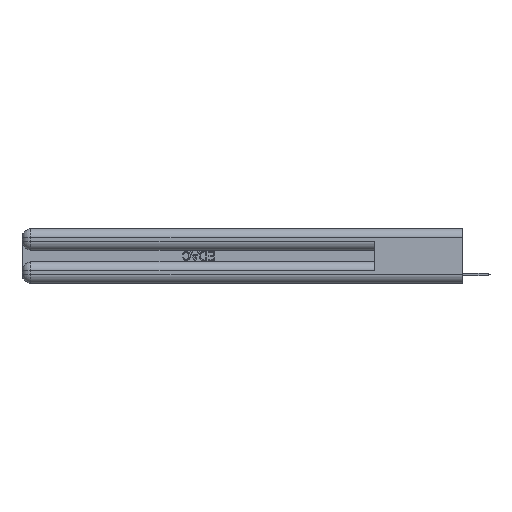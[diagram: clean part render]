
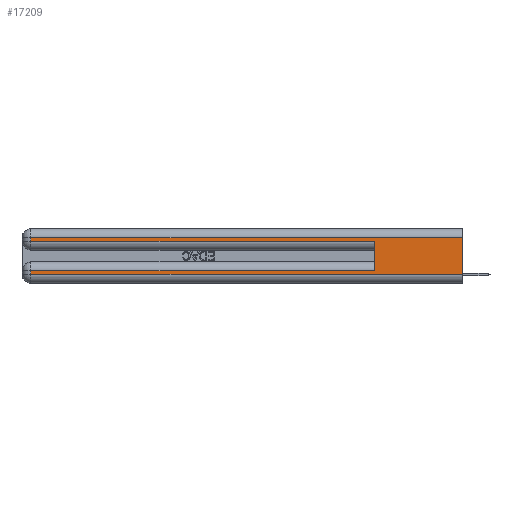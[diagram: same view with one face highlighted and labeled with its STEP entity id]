
A CAD part, left-side view. The second image highlights one B-rep face of the part: STEP entity #17209.
In plain terms, the highlighted planar face has unit normal (-1, 0, 0).
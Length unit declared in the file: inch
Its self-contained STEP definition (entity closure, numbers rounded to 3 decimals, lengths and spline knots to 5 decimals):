
#192 = PLANE ( 'NONE',  #21723 ) ;
#205 = CARTESIAN_POINT ( 'NONE',  ( 0., 2.94, 0.285 ) ) ;
#254 = CARTESIAN_POINT ( 'NONE',  ( 0., 0., 0.37 ) ) ;
#1166 = ORIENTED_EDGE ( 'NONE', *, *, #12571, .T. ) ;
#1764 = CARTESIAN_POINT ( 'NONE',  ( 0., 0., 0.06 ) ) ;
#3998 = ORIENTED_EDGE ( 'NONE', *, *, #26083, .T. ) ;
#4415 = ORIENTED_EDGE ( 'NONE', *, *, #6724, .F. ) ;
#4508 = DIRECTION ( 'NONE',  ( 0., 0., -1. ) ) ;
#4518 = CARTESIAN_POINT ( 'NONE',  ( 0., 2.94, 0.37 ) ) ;
#4592 = DIRECTION ( 'NONE',  ( 0., 0., 1. ) ) ;
#5388 = LINE ( 'NONE', #33290, #15196 ) ;
#5555 = EDGE_CURVE ( 'NONE', #27617, #18806, #10883, .T. ) ;
#5777 = VECTOR ( 'NONE', #33108, 39.37008 ) ;
#6096 = CARTESIAN_POINT ( 'NONE',  ( 0., 2.94, 0.31 ) ) ;
#6724 = EDGE_CURVE ( 'NONE', #21927, #21885, #20685, .T. ) ;
#7761 = DIRECTION ( 'NONE',  ( 0., 1., 0. ) ) ;
#7945 = VECTOR ( 'NONE', #29406, 39.37008 ) ;
#10384 = CARTESIAN_POINT ( 'NONE',  ( 0., 0., 0.31 ) ) ;
#10883 = LINE ( 'NONE', #254, #5777 ) ;
#11114 = CARTESIAN_POINT ( 'NONE',  ( 0., 2.94, 0.06 ) ) ;
#11153 = CARTESIAN_POINT ( 'NONE',  ( 0., 0.6, 0.285 ) ) ;
#12571 = EDGE_CURVE ( 'NONE', #33596, #24471, #13057, .T. ) ;
#13057 = LINE ( 'NONE', #29194, #26706 ) ;
#13869 = CARTESIAN_POINT ( 'NONE',  ( 0., 0., 0.37 ) ) ;
#14155 = LINE ( 'NONE', #4518, #34629 ) ;
#15118 = VECTOR ( 'NONE', #7761, 39.37008 ) ;
#15196 = VECTOR ( 'NONE', #19506, 39.37008 ) ;
#15878 = EDGE_CURVE ( 'NONE', #17169, #18806, #27141, .T. ) ;
#16583 = EDGE_CURVE ( 'NONE', #21927, #20042, #5388, .T. ) ;
#17144 = CARTESIAN_POINT ( 'NONE',  ( 0., 0.6, 0.145 ) ) ;
#17169 = VERTEX_POINT ( 'NONE', #11114 ) ;
#17209 = ADVANCED_FACE ( 'NONE', ( #29239 ), #192, .F. ) ;
#18680 = ORIENTED_EDGE ( 'NONE', *, *, #16583, .T. ) ;
#18706 = EDGE_LOOP ( 'NONE', ( #25665, #3998, #1166, #34211, #4415, #18680, #30239, #34917 ) ) ;
#18806 = VERTEX_POINT ( 'NONE', #27219 ) ;
#19506 = DIRECTION ( 'NONE',  ( 0., 1., 0. ) ) ;
#19569 = VECTOR ( 'NONE', #26799, 39.37008 ) ;
#20042 = VERTEX_POINT ( 'NONE', #34715 ) ;
#20685 = LINE ( 'NONE', #17144, #33932 ) ;
#21189 = DIRECTION ( 'NONE',  ( 0., 0., -1. ) ) ;
#21723 = AXIS2_PLACEMENT_3D ( 'NONE', #13869, #24606, #22079 ) ;
#21885 = VERTEX_POINT ( 'NONE', #11153 ) ;
#21927 = VERTEX_POINT ( 'NONE', #33735 ) ;
#22079 = DIRECTION ( 'NONE',  ( 0., 0., -1. ) ) ;
#24471 = VERTEX_POINT ( 'NONE', #205 ) ;
#24606 = DIRECTION ( 'NONE',  ( 1., 0., 0. ) ) ;
#25665 = ORIENTED_EDGE ( 'NONE', *, *, #5555, .F. ) ;
#26083 = EDGE_CURVE ( 'NONE', #27617, #33596, #30925, .T. ) ;
#26706 = VECTOR ( 'NONE', #4508, 39.37008 ) ;
#26797 = LINE ( 'NONE', #34898, #19569 ) ;
#26799 = DIRECTION ( 'NONE',  ( 0., -1., 0. ) ) ;
#27141 = LINE ( 'NONE', #1764, #7945 ) ;
#27219 = CARTESIAN_POINT ( 'NONE',  ( 0., 0., 0.06 ) ) ;
#27617 = VERTEX_POINT ( 'NONE', #34797 ) ;
#29194 = CARTESIAN_POINT ( 'NONE',  ( 0., 2.94, 0.37 ) ) ;
#29239 = FACE_OUTER_BOUND ( 'NONE', #18706, .T. ) ;
#29406 = DIRECTION ( 'NONE',  ( 0., -1., 0. ) ) ;
#30170 = EDGE_CURVE ( 'NONE', #24471, #21885, #26797, .T. ) ;
#30239 = ORIENTED_EDGE ( 'NONE', *, *, #32179, .T. ) ;
#30925 = LINE ( 'NONE', #10384, #15118 ) ;
#32179 = EDGE_CURVE ( 'NONE', #20042, #17169, #14155, .T. ) ;
#33108 = DIRECTION ( 'NONE',  ( 0., 0., -1. ) ) ;
#33290 = CARTESIAN_POINT ( 'NONE',  ( 0., 0., 0.085 ) ) ;
#33596 = VERTEX_POINT ( 'NONE', #6096 ) ;
#33735 = CARTESIAN_POINT ( 'NONE',  ( 0., 0.6, 0.085 ) ) ;
#33932 = VECTOR ( 'NONE', #4592, 39.37008 ) ;
#34211 = ORIENTED_EDGE ( 'NONE', *, *, #30170, .T. ) ;
#34629 = VECTOR ( 'NONE', #21189, 39.37008 ) ;
#34715 = CARTESIAN_POINT ( 'NONE',  ( 0., 2.94, 0.085 ) ) ;
#34797 = CARTESIAN_POINT ( 'NONE',  ( 0., 0., 0.31 ) ) ;
#34898 = CARTESIAN_POINT ( 'NONE',  ( 0., 0., 0.285 ) ) ;
#34917 = ORIENTED_EDGE ( 'NONE', *, *, #15878, .T. ) ;
